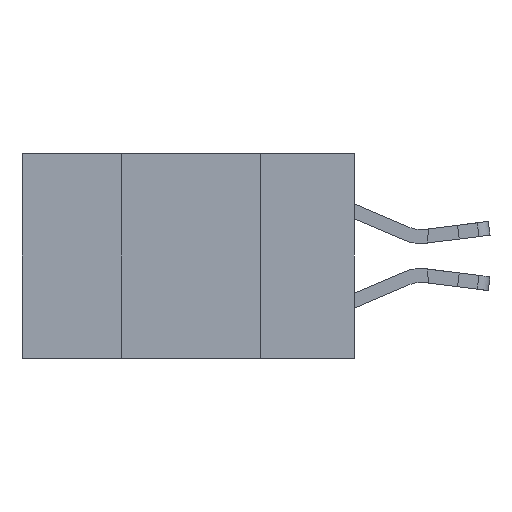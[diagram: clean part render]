
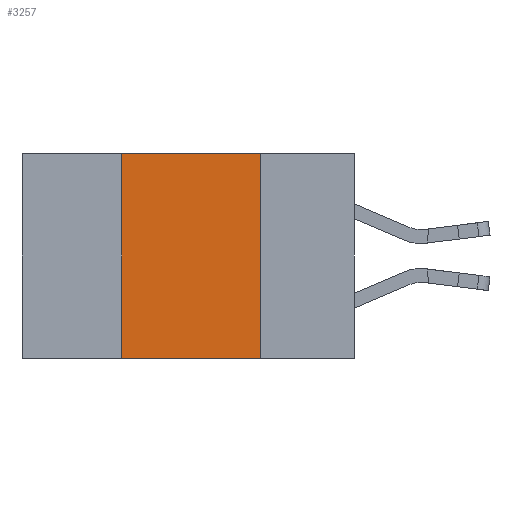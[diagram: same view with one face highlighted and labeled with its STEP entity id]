
A CAD part, left-side view. The second image highlights one B-rep face of the part: STEP entity #3257.
In plain terms, the highlighted planar face has unit normal (-1, 0, 0).
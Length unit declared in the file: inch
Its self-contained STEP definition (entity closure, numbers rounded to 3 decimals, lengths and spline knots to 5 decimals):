
#198 = CARTESIAN_POINT ( 'NONE',  ( 0., 0.17, -0.37 ) ) ;
#502 = VERTEX_POINT ( 'NONE', #8014 ) ;
#556 = CARTESIAN_POINT ( 'NONE',  ( 0., 0.6, -0.37 ) ) ;
#1527 = LINE ( 'NONE', #198, #8047 ) ;
#2209 = EDGE_CURVE ( 'NONE', #5076, #10923, #3023, .T. ) ;
#2506 = ORIENTED_EDGE ( 'NONE', *, *, #5912, .F. ) ;
#2779 = CARTESIAN_POINT ( 'NONE',  ( 0., 0.6, 0. ) ) ;
#2926 = LINE ( 'NONE', #556, #13788 ) ;
#3023 = LINE ( 'NONE', #2779, #15056 ) ;
#3257 = ADVANCED_FACE ( 'NONE', ( #12506 ), #11498, .F. ) ;
#3912 = VECTOR ( 'NONE', #13035, 39.37008 ) ;
#4168 = DIRECTION ( 'NONE',  ( 0., -1., 0. ) ) ;
#4349 = DIRECTION ( 'NONE',  ( 0., -1., 0. ) ) ;
#5076 = VERTEX_POINT ( 'NONE', #14261 ) ;
#5589 = EDGE_LOOP ( 'NONE', ( #12377, #16024, #2506, #14654 ) ) ;
#5912 = EDGE_CURVE ( 'NONE', #9965, #5076, #10342, .T. ) ;
#8014 = CARTESIAN_POINT ( 'NONE',  ( 0., 0.17, -0.37 ) ) ;
#8041 = CARTESIAN_POINT ( 'NONE',  ( 0., 0.42, -0.37 ) ) ;
#8047 = VECTOR ( 'NONE', #12666, 39.37008 ) ;
#8332 = AXIS2_PLACEMENT_3D ( 'NONE', #15124, #9678, #14690 ) ;
#9678 = DIRECTION ( 'NONE',  ( 1., 0., 0. ) ) ;
#9965 = VERTEX_POINT ( 'NONE', #14237 ) ;
#10311 = CARTESIAN_POINT ( 'NONE',  ( 0., 0.17, 0. ) ) ;
#10342 = LINE ( 'NONE', #8041, #3912 ) ;
#10923 = VERTEX_POINT ( 'NONE', #10311 ) ;
#11498 = PLANE ( 'NONE',  #8332 ) ;
#12377 = ORIENTED_EDGE ( 'NONE', *, *, #12637, .F. ) ;
#12461 = EDGE_CURVE ( 'NONE', #9965, #502, #2926, .T. ) ;
#12506 = FACE_OUTER_BOUND ( 'NONE', #5589, .T. ) ;
#12637 = EDGE_CURVE ( 'NONE', #10923, #502, #1527, .T. ) ;
#12666 = DIRECTION ( 'NONE',  ( 0., 0., -1. ) ) ;
#13035 = DIRECTION ( 'NONE',  ( 0., 0., 1. ) ) ;
#13788 = VECTOR ( 'NONE', #4168, 39.37008 ) ;
#14237 = CARTESIAN_POINT ( 'NONE',  ( 0., 0.42, -0.37 ) ) ;
#14261 = CARTESIAN_POINT ( 'NONE',  ( 0., 0.42, 0. ) ) ;
#14654 = ORIENTED_EDGE ( 'NONE', *, *, #12461, .T. ) ;
#14690 = DIRECTION ( 'NONE',  ( 0., 0., -1. ) ) ;
#15056 = VECTOR ( 'NONE', #4349, 39.37008 ) ;
#15124 = CARTESIAN_POINT ( 'NONE',  ( 0., 0.6, 0. ) ) ;
#16024 = ORIENTED_EDGE ( 'NONE', *, *, #2209, .F. ) ;
